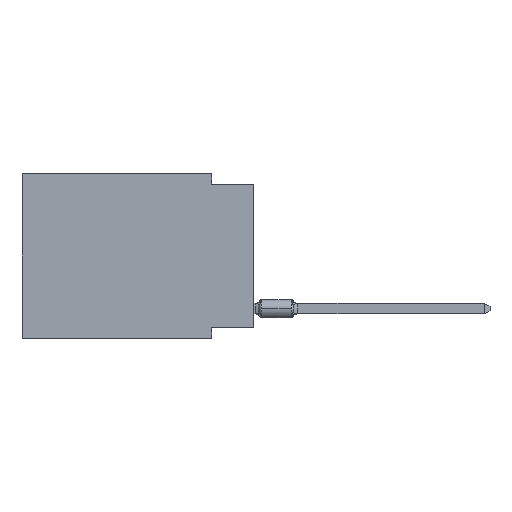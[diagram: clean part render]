
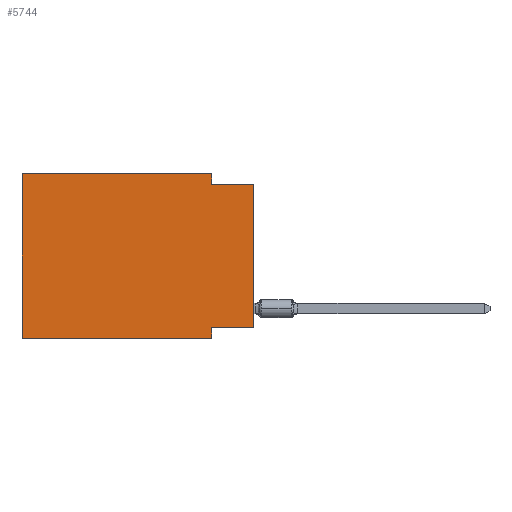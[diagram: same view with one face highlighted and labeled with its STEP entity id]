
A CAD part, left-side view. The second image highlights one B-rep face of the part: STEP entity #5744.
In plain terms, the highlighted planar face has unit normal (-1, 0, 0).
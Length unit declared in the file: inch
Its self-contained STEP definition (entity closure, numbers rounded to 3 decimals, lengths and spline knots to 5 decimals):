
#125 = DIRECTION ( 'NONE',  ( 0., 0., -1. ) ) ;
#172 = EDGE_CURVE ( 'NONE', #7006, #1853, #10775, .T. ) ;
#238 = VERTEX_POINT ( 'NONE', #8431 ) ;
#858 = CARTESIAN_POINT ( 'NONE',  ( 0., 0.1, -0.025 ) ) ;
#895 = ORIENTED_EDGE ( 'NONE', *, *, #172, .F. ) ;
#1116 = VECTOR ( 'NONE', #18330, 39.37008 ) ;
#1853 = VERTEX_POINT ( 'NONE', #3292 ) ;
#2177 = EDGE_CURVE ( 'NONE', #3180, #238, #8357, .T. ) ;
#2252 = CARTESIAN_POINT ( 'NONE',  ( 0., 0.1, 0. ) ) ;
#2612 = ORIENTED_EDGE ( 'NONE', *, *, #11391, .F. ) ;
#3180 = VERTEX_POINT ( 'NONE', #4230 ) ;
#3292 = CARTESIAN_POINT ( 'NONE',  ( 0., 0., -0.025 ) ) ;
#3434 = VERTEX_POINT ( 'NONE', #13235 ) ;
#3489 = EDGE_CURVE ( 'NONE', #9945, #7006, #11862, .T. ) ;
#3669 = DIRECTION ( 'NONE',  ( 0., -1., 0. ) ) ;
#4230 = CARTESIAN_POINT ( 'NONE',  ( 0., 0.55, -0.39 ) ) ;
#4701 = CARTESIAN_POINT ( 'NONE',  ( 0., 0.1, -0.39 ) ) ;
#4728 = EDGE_CURVE ( 'NONE', #238, #9945, #11003, .T. ) ;
#5744 = ADVANCED_FACE ( 'NONE', ( #9809 ), #16271, .F. ) ;
#5778 = ORIENTED_EDGE ( 'NONE', *, *, #2177, .F. ) ;
#6300 = LINE ( 'NONE', #6624, #11602 ) ;
#6624 = CARTESIAN_POINT ( 'NONE',  ( 0., 0., 0. ) ) ;
#6685 = ORIENTED_EDGE ( 'NONE', *, *, #15462, .T. ) ;
#7006 = VERTEX_POINT ( 'NONE', #858 ) ;
#7066 = VECTOR ( 'NONE', #19613, 39.37008 ) ;
#7161 = CARTESIAN_POINT ( 'NONE',  ( 0., 0.1, -0.365 ) ) ;
#7834 = ORIENTED_EDGE ( 'NONE', *, *, #3489, .F. ) ;
#8043 = CARTESIAN_POINT ( 'NONE',  ( 0., 0.55, 0. ) ) ;
#8210 = CARTESIAN_POINT ( 'NONE',  ( 0., 0.55, 0. ) ) ;
#8243 = CARTESIAN_POINT ( 'NONE',  ( 0., 0., -0.365 ) ) ;
#8357 = LINE ( 'NONE', #8043, #7066 ) ;
#8431 = CARTESIAN_POINT ( 'NONE',  ( 0., 0.55, 0. ) ) ;
#9400 = CARTESIAN_POINT ( 'NONE',  ( 0., 0.55, 0. ) ) ;
#9565 = ORIENTED_EDGE ( 'NONE', *, *, #9841, .F. ) ;
#9809 = FACE_OUTER_BOUND ( 'NONE', #18817, .T. ) ;
#9841 = EDGE_CURVE ( 'NONE', #16536, #14208, #17992, .T. ) ;
#9945 = VERTEX_POINT ( 'NONE', #2252 ) ;
#10024 = DIRECTION ( 'NONE',  ( 0., 0., -1. ) ) ;
#10775 = LINE ( 'NONE', #20962, #14889 ) ;
#11003 = LINE ( 'NONE', #9400, #14280 ) ;
#11297 = LINE ( 'NONE', #4701, #19658 ) ;
#11378 = VECTOR ( 'NONE', #18308, 39.37008 ) ;
#11391 = EDGE_CURVE ( 'NONE', #14208, #3434, #11297, .T. ) ;
#11602 = VECTOR ( 'NONE', #19368, 39.37008 ) ;
#11862 = LINE ( 'NONE', #20140, #1116 ) ;
#13235 = CARTESIAN_POINT ( 'NONE',  ( 0., 0.1, -0.39 ) ) ;
#14208 = VERTEX_POINT ( 'NONE', #7161 ) ;
#14280 = VECTOR ( 'NONE', #17461, 39.37008 ) ;
#14289 = VECTOR ( 'NONE', #3669, 39.37008 ) ;
#14675 = DIRECTION ( 'NONE',  ( 1., 0., 0. ) ) ;
#14889 = VECTOR ( 'NONE', #16073, 39.37008 ) ;
#15273 = EDGE_CURVE ( 'NONE', #3180, #3434, #19810, .T. ) ;
#15462 = EDGE_CURVE ( 'NONE', #16536, #1853, #6300, .T. ) ;
#16073 = DIRECTION ( 'NONE',  ( 0., -1., 0. ) ) ;
#16271 = PLANE ( 'NONE',  #20035 ) ;
#16501 = CARTESIAN_POINT ( 'NONE',  ( 0., 0., -0.365 ) ) ;
#16536 = VERTEX_POINT ( 'NONE', #8243 ) ;
#17461 = DIRECTION ( 'NONE',  ( 0., -1., 0. ) ) ;
#17575 = ORIENTED_EDGE ( 'NONE', *, *, #4728, .F. ) ;
#17992 = LINE ( 'NONE', #16501, #11378 ) ;
#18308 = DIRECTION ( 'NONE',  ( 0., 1., 0. ) ) ;
#18330 = DIRECTION ( 'NONE',  ( 0., 0., -1. ) ) ;
#18817 = EDGE_LOOP ( 'NONE', ( #6685, #895, #7834, #17575, #5778, #20185, #2612, #9565 ) ) ;
#19368 = DIRECTION ( 'NONE',  ( 0., 0., 1. ) ) ;
#19613 = DIRECTION ( 'NONE',  ( 0., 0., 1. ) ) ;
#19658 = VECTOR ( 'NONE', #125, 39.37008 ) ;
#19810 = LINE ( 'NONE', #19910, #14289 ) ;
#19910 = CARTESIAN_POINT ( 'NONE',  ( 0., 0.55, -0.39 ) ) ;
#20035 = AXIS2_PLACEMENT_3D ( 'NONE', #8210, #14675, #10024 ) ;
#20140 = CARTESIAN_POINT ( 'NONE',  ( 0., 0.1, 0. ) ) ;
#20185 = ORIENTED_EDGE ( 'NONE', *, *, #15273, .T. ) ;
#20962 = CARTESIAN_POINT ( 'NONE',  ( 0., 0., -0.025 ) ) ;
